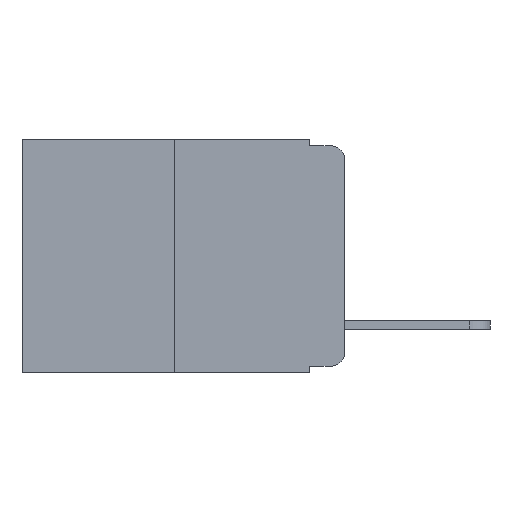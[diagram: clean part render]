
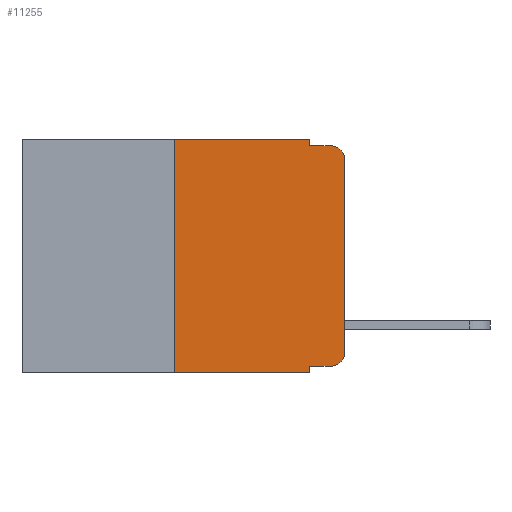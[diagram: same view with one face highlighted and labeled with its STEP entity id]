
A CAD part, left-side view. The second image highlights one B-rep face of the part: STEP entity #11255.
In plain terms, the highlighted planar face has unit normal (-1, 0, 0).
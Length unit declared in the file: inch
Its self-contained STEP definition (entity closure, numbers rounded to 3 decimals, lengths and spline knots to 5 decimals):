
#38 = CARTESIAN_POINT ( 'NONE',  ( 0., 0., -0.03 ) ) ;
#55 = ORIENTED_EDGE ( 'NONE', *, *, #11500, .T. ) ;
#94 = LINE ( 'NONE', #3730, #232 ) ;
#141 = ORIENTED_EDGE ( 'NONE', *, *, #7353, .T. ) ;
#232 = VECTOR ( 'NONE', #967, 39.37008 ) ;
#440 = LINE ( 'NONE', #7281, #493 ) ;
#493 = VECTOR ( 'NONE', #3351, 39.37008 ) ;
#610 = VERTEX_POINT ( 'NONE', #9694 ) ;
#967 = DIRECTION ( 'NONE',  ( 0., -1., 0. ) ) ;
#1225 = VERTEX_POINT ( 'NONE', #6888 ) ;
#1426 = VERTEX_POINT ( 'NONE', #2996 ) ;
#1569 = VECTOR ( 'NONE', #10383, 39.37008 ) ;
#1845 = VECTOR ( 'NONE', #13228, 39.37008 ) ;
#1885 = EDGE_LOOP ( 'NONE', ( #8569, #9311, #9692, #10005, #10722, #7822, #11864, #11943, #141, #55 ) ) ;
#2135 = LINE ( 'NONE', #12057, #1845 ) ;
#2143 = CARTESIAN_POINT ( 'NONE',  ( 0., 0., -0.313 ) ) ;
#2996 = CARTESIAN_POINT ( 'NONE',  ( 0., 0.051, -0.333 ) ) ;
#3139 = VERTEX_POINT ( 'NONE', #3959 ) ;
#3218 = AXIS2_PLACEMENT_3D ( 'NONE', #5984, #5982, #5967 ) ;
#3311 = AXIS2_PLACEMENT_3D ( 'NONE', #9008, #8893, #8881 ) ;
#3351 = DIRECTION ( 'NONE',  ( 0., 0., 1. ) ) ;
#3423 = VERTEX_POINT ( 'NONE', #8010 ) ;
#3455 = VERTEX_POINT ( 'NONE', #6218 ) ;
#3730 = CARTESIAN_POINT ( 'NONE',  ( 0., 0.051, -0.333 ) ) ;
#3847 = LINE ( 'NONE', #6596, #9245 ) ;
#3959 = CARTESIAN_POINT ( 'NONE',  ( 0., 0.25, 0. ) ) ;
#4828 = VERTEX_POINT ( 'NONE', #2143 ) ;
#4920 = AXIS2_PLACEMENT_3D ( 'NONE', #10989, #10959, #10922 ) ;
#5093 = LINE ( 'NONE', #10554, #7541 ) ;
#5119 = CIRCLE ( 'NONE', #3218, 0.02 ) ;
#5967 = DIRECTION ( 'NONE',  ( 0., 0., -1. ) ) ;
#5982 = DIRECTION ( 'NONE',  ( -1., 0., 0. ) ) ;
#5984 = CARTESIAN_POINT ( 'NONE',  ( 0., 0.02, -0.313 ) ) ;
#5999 = EDGE_CURVE ( 'NONE', #4828, #9188, #8712, .T. ) ;
#6218 = CARTESIAN_POINT ( 'NONE',  ( 0., 0.02, -0.333 ) ) ;
#6326 = VERTEX_POINT ( 'NONE', #8203 ) ;
#6554 = DIRECTION ( 'NONE',  ( 0., -1., 0. ) ) ;
#6596 = CARTESIAN_POINT ( 'NONE',  ( 0., 0.473, 0. ) ) ;
#6660 = LINE ( 'NONE', #10180, #8749 ) ;
#6888 = CARTESIAN_POINT ( 'NONE',  ( 0., 0.051, 0. ) ) ;
#6897 = EDGE_CURVE ( 'NONE', #6326, #610, #2135, .T. ) ;
#7234 = EDGE_CURVE ( 'NONE', #6326, #3139, #440, .T. ) ;
#7281 = CARTESIAN_POINT ( 'NONE',  ( 0., 0.25, 0. ) ) ;
#7353 = EDGE_CURVE ( 'NONE', #1426, #3455, #94, .T. ) ;
#7541 = VECTOR ( 'NONE', #10501, 39.37008 ) ;
#7822 = ORIENTED_EDGE ( 'NONE', *, *, #7234, .F. ) ;
#8010 = CARTESIAN_POINT ( 'NONE',  ( 0., 0.02, -0.01 ) ) ;
#8203 = CARTESIAN_POINT ( 'NONE',  ( 0., 0.25, -0.343 ) ) ;
#8244 = CARTESIAN_POINT ( 'NONE',  ( 0., 0.051, -0.01 ) ) ;
#8354 = EDGE_CURVE ( 'NONE', #9188, #3423, #12941, .T. ) ;
#8408 = EDGE_CURVE ( 'NONE', #1225, #8661, #5093, .T. ) ;
#8410 = EDGE_CURVE ( 'NONE', #8661, #3423, #10313, .T. ) ;
#8545 = VECTOR ( 'NONE', #12468, 39.37008 ) ;
#8569 = ORIENTED_EDGE ( 'NONE', *, *, #5999, .T. ) ;
#8661 = VERTEX_POINT ( 'NONE', #8244 ) ;
#8712 = LINE ( 'NONE', #12486, #8545 ) ;
#8749 = VECTOR ( 'NONE', #10205, 39.37008 ) ;
#8881 = DIRECTION ( 'NONE',  ( 0., 0., -1. ) ) ;
#8893 = DIRECTION ( 'NONE',  ( 1., 0., 0. ) ) ;
#8936 = PLANE ( 'NONE',  #3311 ) ;
#9008 = CARTESIAN_POINT ( 'NONE',  ( 0., 0.473, 0. ) ) ;
#9188 = VERTEX_POINT ( 'NONE', #38 ) ;
#9245 = VECTOR ( 'NONE', #6554, 39.37008 ) ;
#9311 = ORIENTED_EDGE ( 'NONE', *, *, #8354, .T. ) ;
#9692 = ORIENTED_EDGE ( 'NONE', *, *, #8410, .F. ) ;
#9694 = CARTESIAN_POINT ( 'NONE',  ( 0., 0.051, -0.343 ) ) ;
#10005 = ORIENTED_EDGE ( 'NONE', *, *, #8408, .F. ) ;
#10180 = CARTESIAN_POINT ( 'NONE',  ( 0., 0.051, 0. ) ) ;
#10205 = DIRECTION ( 'NONE',  ( 0., 0., -1. ) ) ;
#10313 = LINE ( 'NONE', #10460, #1569 ) ;
#10383 = DIRECTION ( 'NONE',  ( 0., -1., 0. ) ) ;
#10460 = CARTESIAN_POINT ( 'NONE',  ( 0., 0.051, -0.01 ) ) ;
#10501 = DIRECTION ( 'NONE',  ( 0., 0., -1. ) ) ;
#10554 = CARTESIAN_POINT ( 'NONE',  ( 0., 0.051, 0. ) ) ;
#10722 = ORIENTED_EDGE ( 'NONE', *, *, #11449, .F. ) ;
#10922 = DIRECTION ( 'NONE',  ( 0., 0., -1. ) ) ;
#10959 = DIRECTION ( 'NONE',  ( -1., 0., 0. ) ) ;
#10989 = CARTESIAN_POINT ( 'NONE',  ( 0., 0.02, -0.03 ) ) ;
#11129 = EDGE_CURVE ( 'NONE', #1426, #610, #6660, .T. ) ;
#11255 = ADVANCED_FACE ( 'NONE', ( #13192 ), #8936, .F. ) ;
#11449 = EDGE_CURVE ( 'NONE', #3139, #1225, #3847, .T. ) ;
#11500 = EDGE_CURVE ( 'NONE', #3455, #4828, #5119, .T. ) ;
#11864 = ORIENTED_EDGE ( 'NONE', *, *, #6897, .T. ) ;
#11943 = ORIENTED_EDGE ( 'NONE', *, *, #11129, .F. ) ;
#12057 = CARTESIAN_POINT ( 'NONE',  ( 0., 0.473, -0.343 ) ) ;
#12468 = DIRECTION ( 'NONE',  ( 0., 0., 1. ) ) ;
#12486 = CARTESIAN_POINT ( 'NONE',  ( 0., 0., 0. ) ) ;
#12941 = CIRCLE ( 'NONE', #4920, 0.02 ) ;
#13192 = FACE_OUTER_BOUND ( 'NONE', #1885, .T. ) ;
#13228 = DIRECTION ( 'NONE',  ( 0., -1., 0. ) ) ;
